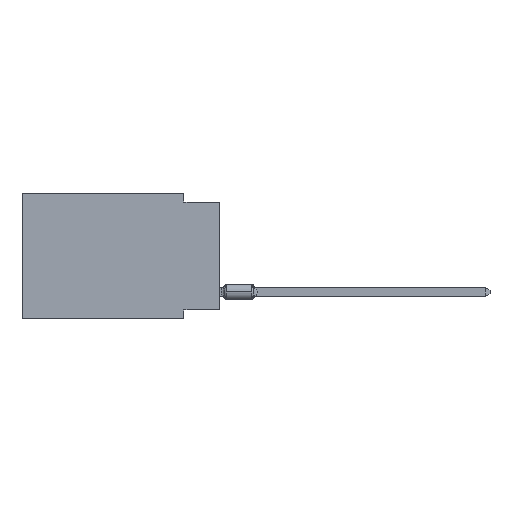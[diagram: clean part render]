
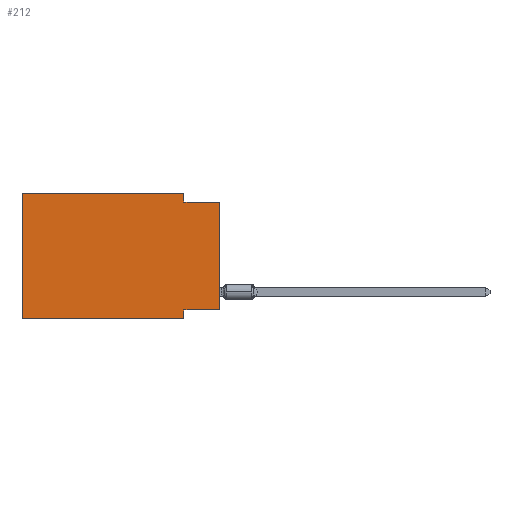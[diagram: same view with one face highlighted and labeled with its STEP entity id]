
A CAD part, left-side view. The second image highlights one B-rep face of the part: STEP entity #212.
In plain terms, the highlighted planar face has unit normal (-1, 0, 0).
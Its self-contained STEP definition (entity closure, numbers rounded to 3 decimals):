
#212 = ADVANCED_FACE ( 'NONE', ( #36787 ), #19318, .F. ) ;
#2666 = CARTESIAN_POINT ( 'NONE',  ( 0., 0., -0.635 ) ) ;
#2848 = DIRECTION ( 'NONE',  ( 0., -1., 0. ) ) ;
#3228 = CARTESIAN_POINT ( 'NONE',  ( 0., 2.54, 0. ) ) ;
#4113 = EDGE_CURVE ( 'NONE', #25270, #6324, #9062, .T. ) ;
#5101 = EDGE_CURVE ( 'NONE', #35161, #24044, #7984, .T. ) ;
#6318 = CARTESIAN_POINT ( 'NONE',  ( 0., 13.97, 0. ) ) ;
#6324 = VERTEX_POINT ( 'NONE', #14922 ) ;
#7101 = CARTESIAN_POINT ( 'NONE',  ( 0., 13.97, -8.89 ) ) ;
#7289 = LINE ( 'NONE', #19032, #30319 ) ;
#7317 = EDGE_LOOP ( 'NONE', ( #20398, #22057, #21609, #17690, #33758, #22640, #20345, #31558 ) ) ;
#7795 = DIRECTION ( 'NONE',  ( 0., 0., -1. ) ) ;
#7984 = LINE ( 'NONE', #28080, #29552 ) ;
#8922 = CARTESIAN_POINT ( 'NONE',  ( 0., 2.54, 0. ) ) ;
#9062 = LINE ( 'NONE', #15319, #15826 ) ;
#9539 = DIRECTION ( 'NONE',  ( 0., -1., 0. ) ) ;
#9623 = DIRECTION ( 'NONE',  ( 0., 0., 1. ) ) ;
#12155 = CARTESIAN_POINT ( 'NONE',  ( 0., 0., -8.255 ) ) ;
#13334 = LINE ( 'NONE', #2666, #33851 ) ;
#13447 = DIRECTION ( 'NONE',  ( 0., 0., -1. ) ) ;
#13691 = EDGE_CURVE ( 'NONE', #6324, #33891, #35531, .T. ) ;
#14053 = EDGE_CURVE ( 'NONE', #14816, #35161, #26378, .T. ) ;
#14059 = CARTESIAN_POINT ( 'NONE',  ( 0., 13.97, -8.89 ) ) ;
#14816 = VERTEX_POINT ( 'NONE', #20172 ) ;
#14922 = CARTESIAN_POINT ( 'NONE',  ( 0., 13.97, 0. ) ) ;
#14991 = DIRECTION ( 'NONE',  ( 0., 1., 0. ) ) ;
#15319 = CARTESIAN_POINT ( 'NONE',  ( 0., 13.97, 0. ) ) ;
#15340 = VERTEX_POINT ( 'NONE', #29410 ) ;
#15689 = DIRECTION ( 'NONE',  ( 0., 0., -1. ) ) ;
#15826 = VECTOR ( 'NONE', #9623, 1000. ) ;
#16564 = CARTESIAN_POINT ( 'NONE',  ( 0., 2.54, -8.89 ) ) ;
#17690 = ORIENTED_EDGE ( 'NONE', *, *, #13691, .F. ) ;
#19032 = CARTESIAN_POINT ( 'NONE',  ( 0., 0., 0. ) ) ;
#19318 = PLANE ( 'NONE',  #36309 ) ;
#19407 = DIRECTION ( 'NONE',  ( 0., 0., 1. ) ) ;
#19524 = CARTESIAN_POINT ( 'NONE',  ( 0., 0., -0.635 ) ) ;
#20172 = CARTESIAN_POINT ( 'NONE',  ( 0., 0., -8.255 ) ) ;
#20345 = ORIENTED_EDGE ( 'NONE', *, *, #5101, .F. ) ;
#20398 = ORIENTED_EDGE ( 'NONE', *, *, #34358, .T. ) ;
#21609 = ORIENTED_EDGE ( 'NONE', *, *, #23497, .F. ) ;
#21782 = VECTOR ( 'NONE', #28120, 1000. ) ;
#22057 = ORIENTED_EDGE ( 'NONE', *, *, #32560, .F. ) ;
#22329 = VECTOR ( 'NONE', #15689, 1000. ) ;
#22640 = ORIENTED_EDGE ( 'NONE', *, *, #33168, .T. ) ;
#23221 = VECTOR ( 'NONE', #14991, 1000. ) ;
#23497 = EDGE_CURVE ( 'NONE', #33891, #15340, #29202, .T. ) ;
#24044 = VERTEX_POINT ( 'NONE', #16564 ) ;
#24452 = CARTESIAN_POINT ( 'NONE',  ( 0., 13.97, 0. ) ) ;
#24821 = CARTESIAN_POINT ( 'NONE',  ( 0., 2.54, -8.255 ) ) ;
#24822 = DIRECTION ( 'NONE',  ( 1., 0., 0. ) ) ;
#25270 = VERTEX_POINT ( 'NONE', #14059 ) ;
#26378 = LINE ( 'NONE', #12155, #23221 ) ;
#28080 = CARTESIAN_POINT ( 'NONE',  ( 0., 2.54, -8.89 ) ) ;
#28120 = DIRECTION ( 'NONE',  ( 0., -1., 0. ) ) ;
#29202 = LINE ( 'NONE', #3228, #22329 ) ;
#29410 = CARTESIAN_POINT ( 'NONE',  ( 0., 2.54, -0.635 ) ) ;
#29552 = VECTOR ( 'NONE', #7795, 1000. ) ;
#30221 = VERTEX_POINT ( 'NONE', #19524 ) ;
#30319 = VECTOR ( 'NONE', #19407, 1000. ) ;
#31558 = ORIENTED_EDGE ( 'NONE', *, *, #14053, .F. ) ;
#32560 = EDGE_CURVE ( 'NONE', #15340, #30221, #13334, .T. ) ;
#33168 = EDGE_CURVE ( 'NONE', #25270, #24044, #36681, .T. ) ;
#33493 = VECTOR ( 'NONE', #9539, 1000. ) ;
#33758 = ORIENTED_EDGE ( 'NONE', *, *, #4113, .F. ) ;
#33851 = VECTOR ( 'NONE', #2848, 1000. ) ;
#33891 = VERTEX_POINT ( 'NONE', #8922 ) ;
#34358 = EDGE_CURVE ( 'NONE', #14816, #30221, #7289, .T. ) ;
#35161 = VERTEX_POINT ( 'NONE', #24821 ) ;
#35531 = LINE ( 'NONE', #6318, #33493 ) ;
#36309 = AXIS2_PLACEMENT_3D ( 'NONE', #24452, #24822, #13447 ) ;
#36681 = LINE ( 'NONE', #7101, #21782 ) ;
#36787 = FACE_OUTER_BOUND ( 'NONE', #7317, .T. ) ;
